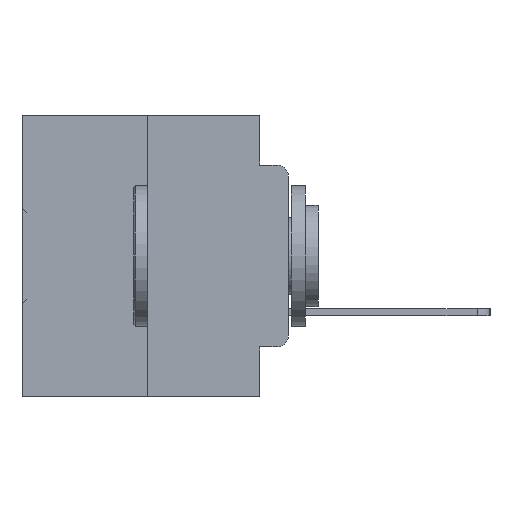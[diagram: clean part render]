
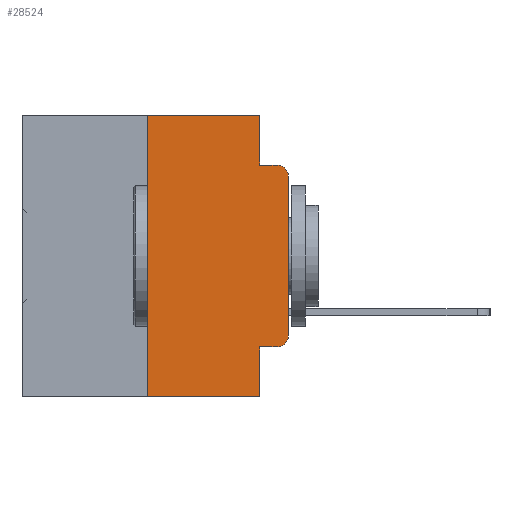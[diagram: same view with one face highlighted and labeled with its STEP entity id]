
A CAD part, left-side view. The second image highlights one B-rep face of the part: STEP entity #28524.
In plain terms, the highlighted planar face has unit normal (-1, 0, 0).
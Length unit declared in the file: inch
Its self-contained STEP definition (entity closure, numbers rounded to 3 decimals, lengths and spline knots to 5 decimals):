
#267 = CARTESIAN_POINT ( 'NONE',  ( 0., 0.02, -0.0885 ) ) ;
#322 = AXIS2_PLACEMENT_3D ( 'NONE', #19585, #9286, #27456 ) ;
#1468 = ORIENTED_EDGE ( 'NONE', *, *, #22808, .F. ) ;
#1957 = EDGE_LOOP ( 'NONE', ( #10174, #15117, #2656, #6845, #30086, #1468, #9398, #11075, #16771, #4392 ) ) ;
#2619 = EDGE_CURVE ( 'NONE', #3305, #11722, #33056, .T. ) ;
#2656 = ORIENTED_EDGE ( 'NONE', *, *, #2619, .F. ) ;
#2677 = LINE ( 'NONE', #33593, #16745 ) ;
#3305 = VERTEX_POINT ( 'NONE', #24096 ) ;
#3792 = VERTEX_POINT ( 'NONE', #25832 ) ;
#3914 = PLANE ( 'NONE',  #322 ) ;
#4090 = DIRECTION ( 'NONE',  ( 0., 0., -1. ) ) ;
#4392 = ORIENTED_EDGE ( 'NONE', *, *, #7372, .T. ) ;
#4690 = VERTEX_POINT ( 'NONE', #14399 ) ;
#4809 = VERTEX_POINT ( 'NONE', #25639 ) ;
#5094 = CARTESIAN_POINT ( 'NONE',  ( 0., 0.051, -0.0885 ) ) ;
#6079 = EDGE_CURVE ( 'NONE', #11882, #4809, #2677, .T. ) ;
#6396 = EDGE_CURVE ( 'NONE', #9065, #4690, #22223, .T. ) ;
#6845 = ORIENTED_EDGE ( 'NONE', *, *, #31720, .F. ) ;
#6905 = EDGE_CURVE ( 'NONE', #29307, #23408, #22639, .T. ) ;
#7372 = EDGE_CURVE ( 'NONE', #23408, #9065, #17408, .T. ) ;
#7759 = DIRECTION ( 'NONE',  ( 0., -1., 0. ) ) ;
#8414 = VECTOR ( 'NONE', #11427, 39.37008 ) ;
#8772 = CARTESIAN_POINT ( 'NONE',  ( 0., 0., 0. ) ) ;
#8791 = VECTOR ( 'NONE', #4090, 39.37008 ) ;
#8931 = CARTESIAN_POINT ( 'NONE',  ( 0., 0.25, 0. ) ) ;
#9065 = VERTEX_POINT ( 'NONE', #17162 ) ;
#9286 = DIRECTION ( 'NONE',  ( 1., 0., 0. ) ) ;
#9398 = ORIENTED_EDGE ( 'NONE', *, *, #17135, .T. ) ;
#10174 = ORIENTED_EDGE ( 'NONE', *, *, #6396, .T. ) ;
#10446 = EDGE_CURVE ( 'NONE', #4690, #11722, #13920, .T. ) ;
#11075 = ORIENTED_EDGE ( 'NONE', *, *, #14695, .F. ) ;
#11218 = CARTESIAN_POINT ( 'NONE',  ( 0., 0.473, -0.5 ) ) ;
#11427 = DIRECTION ( 'NONE',  ( 0., 0., 1. ) ) ;
#11561 = VECTOR ( 'NONE', #33338, 39.37008 ) ;
#11722 = VERTEX_POINT ( 'NONE', #267 ) ;
#11882 = VERTEX_POINT ( 'NONE', #8931 ) ;
#12743 = CARTESIAN_POINT ( 'NONE',  ( 0., 0.02, -0.1085 ) ) ;
#13538 = LINE ( 'NONE', #29621, #32462 ) ;
#13920 = CIRCLE ( 'NONE', #14787, 0.02 ) ;
#14399 = CARTESIAN_POINT ( 'NONE',  ( 0., 0., -0.1085 ) ) ;
#14682 = CARTESIAN_POINT ( 'NONE',  ( 0., 0.051, 0. ) ) ;
#14695 = EDGE_CURVE ( 'NONE', #29307, #3792, #33781, .T. ) ;
#14787 = AXIS2_PLACEMENT_3D ( 'NONE', #12743, #30828, #15378 ) ;
#15117 = ORIENTED_EDGE ( 'NONE', *, *, #10446, .T. ) ;
#15125 = CARTESIAN_POINT ( 'NONE',  ( 0., 0.02, -0.3915 ) ) ;
#15378 = DIRECTION ( 'NONE',  ( 0., 0., -1. ) ) ;
#15816 = LINE ( 'NONE', #14682, #8791 ) ;
#16745 = VECTOR ( 'NONE', #31042, 39.37008 ) ;
#16771 = ORIENTED_EDGE ( 'NONE', *, *, #6905, .T. ) ;
#17135 = EDGE_CURVE ( 'NONE', #19042, #3792, #25918, .T. ) ;
#17162 = CARTESIAN_POINT ( 'NONE',  ( 0., 0., -0.3915 ) ) ;
#17408 = CIRCLE ( 'NONE', #19405, 0.02 ) ;
#17667 = DIRECTION ( 'NONE',  ( 0., 0., -1. ) ) ;
#17911 = CARTESIAN_POINT ( 'NONE',  ( 0., 0.25, -0.5 ) ) ;
#18713 = CARTESIAN_POINT ( 'NONE',  ( 0., 0.051, -0.4115 ) ) ;
#19007 = DIRECTION ( 'NONE',  ( 0., -1., 0. ) ) ;
#19042 = VERTEX_POINT ( 'NONE', #17911 ) ;
#19405 = AXIS2_PLACEMENT_3D ( 'NONE', #15125, #33130, #17667 ) ;
#19585 = CARTESIAN_POINT ( 'NONE',  ( 0., 0.473, 0. ) ) ;
#21988 = CARTESIAN_POINT ( 'NONE',  ( 0., 0.02, -0.4115 ) ) ;
#22223 = LINE ( 'NONE', #8772, #8414 ) ;
#22639 = LINE ( 'NONE', #18713, #28795 ) ;
#22808 = EDGE_CURVE ( 'NONE', #19042, #11882, #13538, .T. ) ;
#22942 = CARTESIAN_POINT ( 'NONE',  ( 0., 0.051, -0.4115 ) ) ;
#23408 = VERTEX_POINT ( 'NONE', #21988 ) ;
#24096 = CARTESIAN_POINT ( 'NONE',  ( 0., 0.051, -0.0885 ) ) ;
#25639 = CARTESIAN_POINT ( 'NONE',  ( 0., 0.051, 0. ) ) ;
#25832 = CARTESIAN_POINT ( 'NONE',  ( 0., 0.051, -0.5 ) ) ;
#25918 = LINE ( 'NONE', #11218, #31953 ) ;
#27320 = FACE_OUTER_BOUND ( 'NONE', #1957, .T. ) ;
#27456 = DIRECTION ( 'NONE',  ( 0., 0., -1. ) ) ;
#28524 = ADVANCED_FACE ( 'NONE', ( #27320 ), #3914, .F. ) ;
#28795 = VECTOR ( 'NONE', #29056, 39.37008 ) ;
#29056 = DIRECTION ( 'NONE',  ( 0., -1., 0. ) ) ;
#29307 = VERTEX_POINT ( 'NONE', #22942 ) ;
#29621 = CARTESIAN_POINT ( 'NONE',  ( 0., 0.25, 0. ) ) ;
#30086 = ORIENTED_EDGE ( 'NONE', *, *, #6079, .F. ) ;
#30814 = CARTESIAN_POINT ( 'NONE',  ( 0., 0.051, 0. ) ) ;
#30828 = DIRECTION ( 'NONE',  ( -1., 0., 0. ) ) ;
#31042 = DIRECTION ( 'NONE',  ( 0., -1., 0. ) ) ;
#31720 = EDGE_CURVE ( 'NONE', #4809, #3305, #15816, .T. ) ;
#31953 = VECTOR ( 'NONE', #19007, 39.37008 ) ;
#32158 = DIRECTION ( 'NONE',  ( 0., 0., 1. ) ) ;
#32264 = VECTOR ( 'NONE', #7759, 39.37008 ) ;
#32462 = VECTOR ( 'NONE', #32158, 39.37008 ) ;
#33056 = LINE ( 'NONE', #5094, #32264 ) ;
#33130 = DIRECTION ( 'NONE',  ( -1., 0., 0. ) ) ;
#33338 = DIRECTION ( 'NONE',  ( 0., 0., -1. ) ) ;
#33593 = CARTESIAN_POINT ( 'NONE',  ( 0., 0.473, 0. ) ) ;
#33781 = LINE ( 'NONE', #30814, #11561 ) ;
